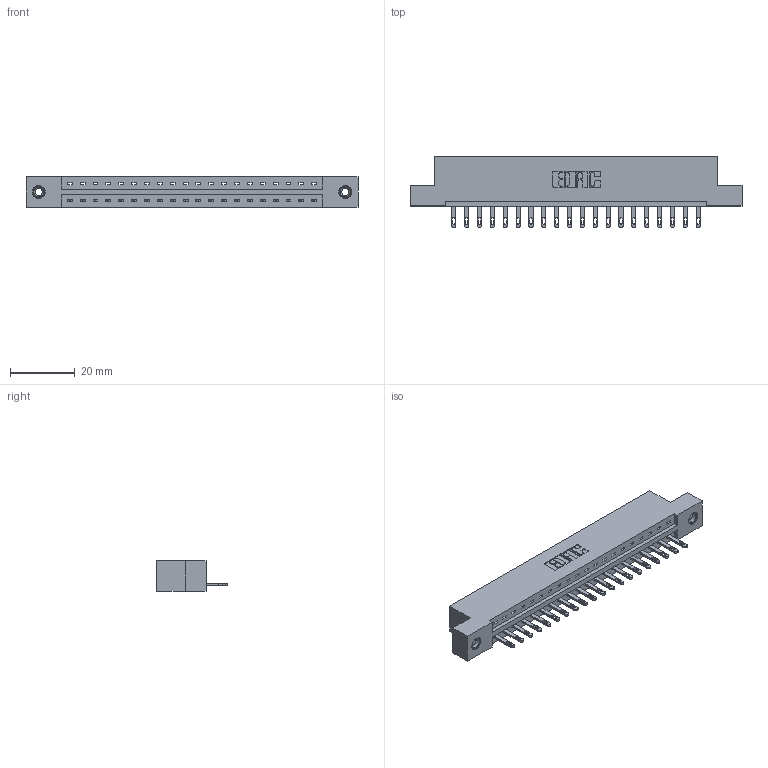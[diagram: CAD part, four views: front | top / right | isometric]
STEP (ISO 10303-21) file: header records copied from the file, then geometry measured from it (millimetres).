
FILE_DESCRIPTION (( 'STEP AP203' ), '1' );
FILE_NAME ('887-020-500-108.STEP', '2020-09-20T18:04:44', ( '' ), ( '' ), 'SwSTEP 2.0', 'SolidWorks 2020', '' );
FILE_SCHEMA (( 'CONFIG_CONTROL_DESIGN' ));
Length unit declared in the file: inch
Products named in the file (4): 887-020-500-108; 345-250-001_345-250-003-102; 345-292-001_345-293-100; 837 Part_Flush Mounting Lugs - 0.156 Dia-TI
Assembly tree (23 placements, depth 2):
  887-020-500-108
    837 Part_Flush Mounting Lugs - 0.156 Dia-TI
    345-292-001_345-293-100  x20
    345-250-001_345-250-003-102  x2
Bounding box: 102.26 x 21.85 x 9.4 mm (x, y, z)
Volume: 10358.8 mm3; surface area: 10658.6 mm2
Topology: 23 solids, 23 shells, 1334 faces, 4047 edges, 2690 vertices
Faces by surface type: plane 902, cylinder 416, cone 12, torus 4
Entity records: 18828 total; most frequent: CARTESIAN_POINT 3257, ORIENTED_EDGE 3206, DIRECTION 2821, EDGE_CURVE 1603, VECTOR 1451, LINE 1451, VERTEX_POINT 1064, AXIS2_PLACEMENT_3D 685
